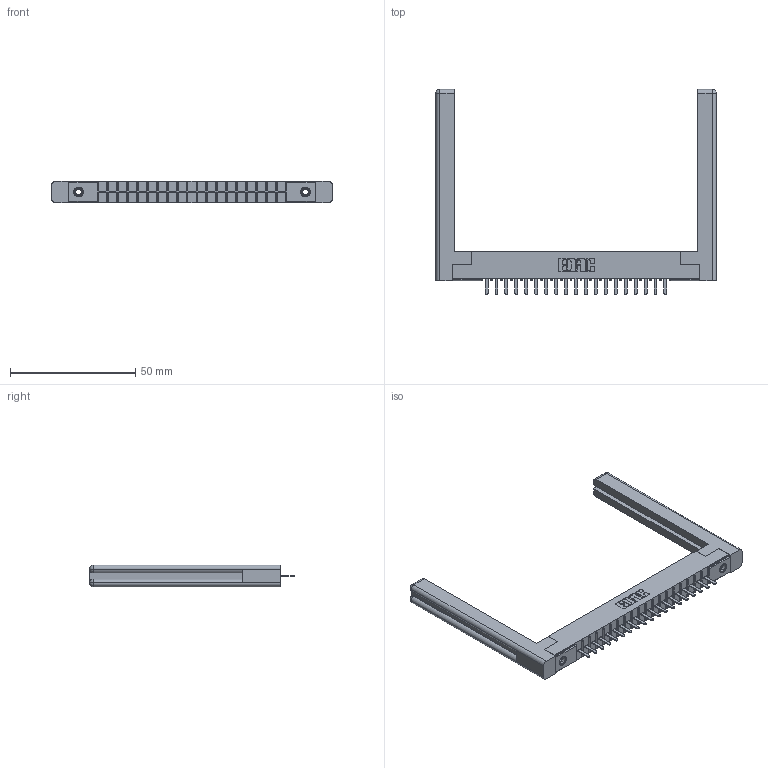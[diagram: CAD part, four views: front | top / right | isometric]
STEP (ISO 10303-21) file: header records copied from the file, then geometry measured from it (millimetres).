
FILE_DESCRIPTION (( 'STEP AP203' ), '1' );
FILE_NAME ('306-019-420-158.STEP', '2020-09-21T20:01:58', ( '' ), ( '' ), 'SwSTEP 2.0', 'SolidWorks 2020', '' );
FILE_SCHEMA (( 'CONFIG_CONTROL_DESIGN' ));
Length unit declared in the file: inch
Products named in the file (5): 345-250-001_345-250-001-102; 306-290-001_120; 306-019-420-158; 307-220-058; 306 Part_.156 Dia
Assembly tree (24 placements, depth 2):
  306-019-420-158
    306 Part_.156 Dia
    306-290-001_120  x19
    345-250-001_345-250-001-102  x2
    307-220-058  x2
Bounding box: 111.91 x 81.76 x 8.71 mm (x, y, z)
Volume: 15285.5 mm3; surface area: 16502.6 mm2
Topology: 24 solids, 24 shells, 1588 faces, 4413 edges, 2826 vertices
Faces by surface type: plane 1045, cylinder 443, sphere 76, cone 12, torus 12
Entity records: 23287 total; most frequent: CARTESIAN_POINT 3915, ORIENTED_EDGE 3820, DIRECTION 3818, EDGE_CURVE 1910, VECTOR 1476, LINE 1476, VERTEX_POINT 1214, AXIS2_PLACEMENT_3D 1171
